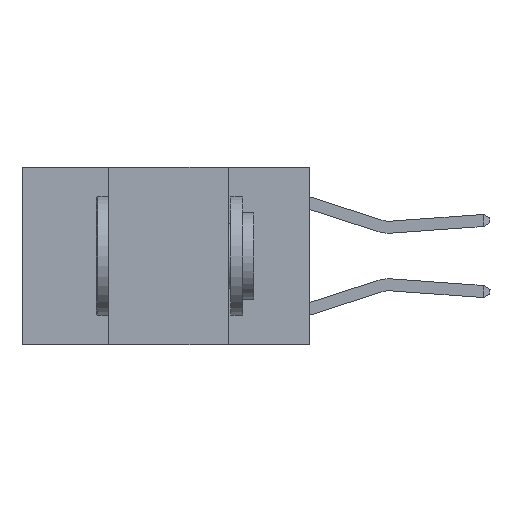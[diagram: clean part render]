
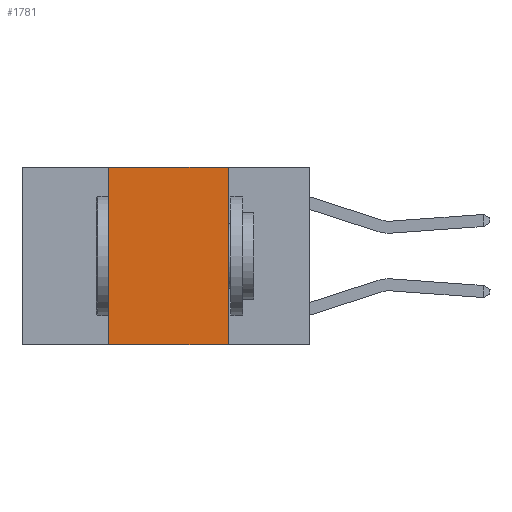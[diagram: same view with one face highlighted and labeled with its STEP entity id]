
A CAD part, left-side view. The second image highlights one B-rep face of the part: STEP entity #1781.
In plain terms, the highlighted planar face has unit normal (-1, 0, 0).
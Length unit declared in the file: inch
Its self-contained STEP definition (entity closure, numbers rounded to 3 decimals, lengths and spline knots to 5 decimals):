
#357 = DIRECTION ( 'NONE',  ( 0., 0., 1. ) ) ;
#1006 = EDGE_CURVE ( 'NONE', #14886, #14822, #1845, .T. ) ;
#1197 = LINE ( 'NONE', #7008, #10718 ) ;
#1727 = EDGE_LOOP ( 'NONE', ( #7805, #6274, #15387, #15202 ) ) ;
#1781 = ADVANCED_FACE ( 'NONE', ( #17141 ), #7250, .F. ) ;
#1845 = LINE ( 'NONE', #14872, #11866 ) ;
#3344 = AXIS2_PLACEMENT_3D ( 'NONE', #9932, #17336, #4203 ) ;
#3873 = CARTESIAN_POINT ( 'NONE',  ( 0., 0.6, 0. ) ) ;
#4137 = CARTESIAN_POINT ( 'NONE',  ( 0., 0.42, -0.37 ) ) ;
#4203 = DIRECTION ( 'NONE',  ( 0., 0., -1. ) ) ;
#4998 = VECTOR ( 'NONE', #16913, 39.37008 ) ;
#5590 = CARTESIAN_POINT ( 'NONE',  ( 0., 0.17, 0. ) ) ;
#6274 = ORIENTED_EDGE ( 'NONE', *, *, #13027, .F. ) ;
#6707 = CARTESIAN_POINT ( 'NONE',  ( 0., 0.17, -0.37 ) ) ;
#7008 = CARTESIAN_POINT ( 'NONE',  ( 0., 0.6, -0.37 ) ) ;
#7250 = PLANE ( 'NONE',  #3344 ) ;
#7662 = VERTEX_POINT ( 'NONE', #5590 ) ;
#7805 = ORIENTED_EDGE ( 'NONE', *, *, #16981, .F. ) ;
#9670 = CARTESIAN_POINT ( 'NONE',  ( 0., 0.17, 0. ) ) ;
#9932 = CARTESIAN_POINT ( 'NONE',  ( 0., 0.6, 0. ) ) ;
#10482 = EDGE_CURVE ( 'NONE', #14886, #16945, #1197, .T. ) ;
#10718 = VECTOR ( 'NONE', #14495, 39.37008 ) ;
#11866 = VECTOR ( 'NONE', #357, 39.37008 ) ;
#12559 = DIRECTION ( 'NONE',  ( 0., 0., -1. ) ) ;
#12659 = CARTESIAN_POINT ( 'NONE',  ( 0., 0.42, 0. ) ) ;
#13027 = EDGE_CURVE ( 'NONE', #14822, #7662, #16998, .T. ) ;
#13363 = VECTOR ( 'NONE', #12559, 39.37008 ) ;
#14495 = DIRECTION ( 'NONE',  ( 0., -1., 0. ) ) ;
#14822 = VERTEX_POINT ( 'NONE', #12659 ) ;
#14872 = CARTESIAN_POINT ( 'NONE',  ( 0., 0.42, 0. ) ) ;
#14886 = VERTEX_POINT ( 'NONE', #4137 ) ;
#15202 = ORIENTED_EDGE ( 'NONE', *, *, #10482, .T. ) ;
#15387 = ORIENTED_EDGE ( 'NONE', *, *, #1006, .F. ) ;
#16913 = DIRECTION ( 'NONE',  ( 0., -1., 0. ) ) ;
#16945 = VERTEX_POINT ( 'NONE', #6707 ) ;
#16981 = EDGE_CURVE ( 'NONE', #7662, #16945, #18698, .T. ) ;
#16998 = LINE ( 'NONE', #3873, #4998 ) ;
#17141 = FACE_OUTER_BOUND ( 'NONE', #1727, .T. ) ;
#17336 = DIRECTION ( 'NONE',  ( 1., 0., 0. ) ) ;
#18698 = LINE ( 'NONE', #9670, #13363 ) ;
